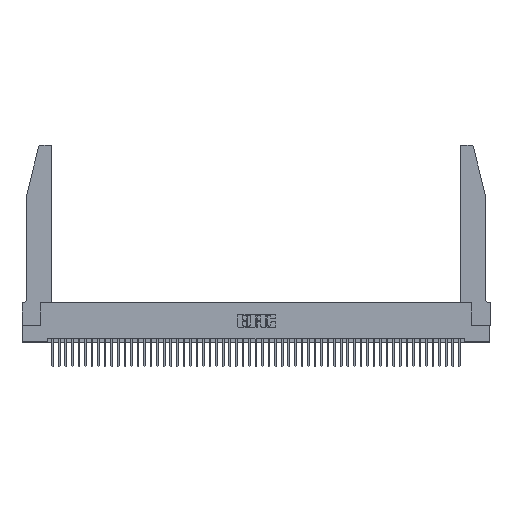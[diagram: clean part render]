
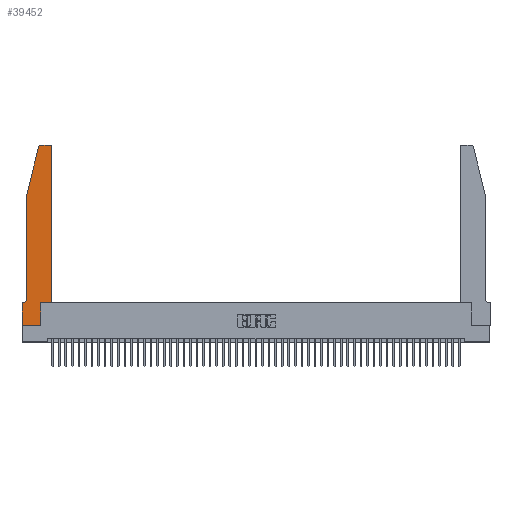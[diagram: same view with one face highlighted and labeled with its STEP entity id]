
A CAD part, top view. The second image highlights one B-rep face of the part: STEP entity #39452.
In plain terms, the highlighted planar face has unit normal (0, 0, 1).
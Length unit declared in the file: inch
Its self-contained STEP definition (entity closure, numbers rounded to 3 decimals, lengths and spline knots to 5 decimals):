
#424 = LINE ( 'NONE', #24426, #38902 ) ;
#468 = VECTOR ( 'NONE', #25666, 39.37008 ) ;
#502 = AXIS2_PLACEMENT_3D ( 'NONE', #27071, #50351, #46513 ) ;
#571 = VERTEX_POINT ( 'NONE', #48811 ) ;
#1234 = CARTESIAN_POINT ( 'NONE',  ( 0.2605, 2.75, 0.37 ) ) ;
#1330 = VECTOR ( 'NONE', #19724, 39.37008 ) ;
#1846 = DIRECTION ( 'NONE',  ( 0., -1., 0. ) ) ;
#2422 = EDGE_CURVE ( 'NONE', #31493, #47907, #22815, .T. ) ;
#2819 = VECTOR ( 'NONE', #23073, 39.37008 ) ;
#2908 = CARTESIAN_POINT ( 'NONE',  ( 0., 0., 0.37 ) ) ;
#2964 = ORIENTED_EDGE ( 'NONE', *, *, #2422, .T. ) ;
#2999 = EDGE_CURVE ( 'NONE', #46961, #31018, #424, .T. ) ;
#3189 = CARTESIAN_POINT ( 'NONE',  ( 0.284, 2.75, 0.37 ) ) ;
#3436 = CARTESIAN_POINT ( 'NONE',  ( 0.2865, 0.35, 0.37 ) ) ;
#4125 = CIRCLE ( 'NONE', #18013, 0.03 ) ;
#4364 = CIRCLE ( 'NONE', #39853, 0.03 ) ;
#5432 = ORIENTED_EDGE ( 'NONE', *, *, #38660, .T. ) ;
#5646 = EDGE_CURVE ( 'NONE', #20788, #46961, #23670, .T. ) ;
#6351 = VECTOR ( 'NONE', #25296, 39.37008 ) ;
#6635 = PLANE ( 'NONE',  #33865 ) ;
#7294 = CARTESIAN_POINT ( 'NONE',  ( 0.0055, 0.35, 0.37 ) ) ;
#7648 = VECTOR ( 'NONE', #30325, 39.37008 ) ;
#7833 = ORIENTED_EDGE ( 'NONE', *, *, #25196, .T. ) ;
#7897 = ORIENTED_EDGE ( 'NONE', *, *, #5646, .T. ) ;
#8317 = CARTESIAN_POINT ( 'NONE',  ( 0.2865, 0.35, 0.37 ) ) ;
#9077 = ORIENTED_EDGE ( 'NONE', *, *, #36775, .T. ) ;
#9507 = EDGE_CURVE ( 'NONE', #31018, #13375, #33835, .T. ) ;
#9522 = CARTESIAN_POINT ( 'NONE',  ( 0.0755, 2., 0.37 ) ) ;
#10010 = ORIENTED_EDGE ( 'NONE', *, *, #2999, .T. ) ;
#10829 = CARTESIAN_POINT ( 'NONE',  ( 0., 0.35, 0.37 ) ) ;
#11681 = VERTEX_POINT ( 'NONE', #48966 ) ;
#11973 = VERTEX_POINT ( 'NONE', #2908 ) ;
#12376 = ORIENTED_EDGE ( 'NONE', *, *, #41454, .T. ) ;
#13375 = VERTEX_POINT ( 'NONE', #30405 ) ;
#13486 = ORIENTED_EDGE ( 'NONE', *, *, #9507, .T. ) ;
#14643 = DIRECTION ( 'NONE',  ( 1., 0., 0. ) ) ;
#15392 = ORIENTED_EDGE ( 'NONE', *, *, #37172, .T. ) ;
#15480 = CARTESIAN_POINT ( 'NONE',  ( 0.284, 2.72, 0.37 ) ) ;
#15869 = CARTESIAN_POINT ( 'NONE',  ( 0., 0., 0.37 ) ) ;
#16995 = DIRECTION ( 'NONE',  ( 1., 0., 0. ) ) ;
#18013 = AXIS2_PLACEMENT_3D ( 'NONE', #24133, #36294, #28321 ) ;
#18728 = VERTEX_POINT ( 'NONE', #3189 ) ;
#19566 = VECTOR ( 'NONE', #28675, 39.37008 ) ;
#19724 = DIRECTION ( 'NONE',  ( 0., 1., 0. ) ) ;
#20788 = VERTEX_POINT ( 'NONE', #32162 ) ;
#21503 = CARTESIAN_POINT ( 'NONE',  ( 0.0755, 2., 0.37 ) ) ;
#21998 = CARTESIAN_POINT ( 'NONE',  ( 0.25487, 2.72718, 0.37 ) ) ;
#22579 = DIRECTION ( 'NONE',  ( 0., 0., 1. ) ) ;
#22815 = LINE ( 'NONE', #21503, #468 ) ;
#23073 = DIRECTION ( 'NONE',  ( 0., 1., 0. ) ) ;
#23145 = LINE ( 'NONE', #50287, #7648 ) ;
#23670 = LINE ( 'NONE', #8317, #1330 ) ;
#23831 = CARTESIAN_POINT ( 'NONE',  ( 0., 0.35, 0.37 ) ) ;
#24133 = CARTESIAN_POINT ( 'NONE',  ( 0.4205, 2.72, 0.37 ) ) ;
#24426 = CARTESIAN_POINT ( 'NONE',  ( 0.4505, 0.35, 0.37 ) ) ;
#24774 = ORIENTED_EDGE ( 'NONE', *, *, #33399, .T. ) ;
#24796 = VECTOR ( 'NONE', #1846, 39.37008 ) ;
#25196 = EDGE_CURVE ( 'NONE', #18728, #31493, #4364, .T. ) ;
#25296 = DIRECTION ( 'NONE',  ( 1., 0., 0. ) ) ;
#25666 = DIRECTION ( 'NONE',  ( -0.239, -0.971, 0. ) ) ;
#26063 = EDGE_LOOP ( 'NONE', ( #12376, #7833, #2964, #5432, #48761, #9077, #15392, #24774, #7897, #10010, #13486, #45482 ) ) ;
#26932 = DIRECTION ( 'NONE',  ( 0., 0., 1. ) ) ;
#27071 = CARTESIAN_POINT ( 'NONE',  ( 0.0055, 0.42, 0.37 ) ) ;
#27257 = CARTESIAN_POINT ( 'NONE',  ( 0.4505, 0.35, 0.37 ) ) ;
#28321 = DIRECTION ( 'NONE',  ( 1., 0., 0. ) ) ;
#28675 = DIRECTION ( 'NONE',  ( -1., 0., 0. ) ) ;
#29334 = VERTEX_POINT ( 'NONE', #7294 ) ;
#30163 = LINE ( 'NONE', #1234, #19566 ) ;
#30297 = FACE_OUTER_BOUND ( 'NONE', #26063, .T. ) ;
#30325 = DIRECTION ( 'NONE',  ( -1., 0., 0. ) ) ;
#30405 = CARTESIAN_POINT ( 'NONE',  ( 0.4505, 2.72, 0.37 ) ) ;
#30602 = VECTOR ( 'NONE', #51102, 39.37008 ) ;
#31018 = VERTEX_POINT ( 'NONE', #50860 ) ;
#31493 = VERTEX_POINT ( 'NONE', #21998 ) ;
#32162 = CARTESIAN_POINT ( 'NONE',  ( 0.2865, 0., 0.37 ) ) ;
#32775 = CIRCLE ( 'NONE', #502, 0.07 ) ;
#33399 = EDGE_CURVE ( 'NONE', #11973, #20788, #43574, .T. ) ;
#33442 = CARTESIAN_POINT ( 'NONE',  ( 0., 0., 0.37 ) ) ;
#33835 = LINE ( 'NONE', #27257, #2819 ) ;
#33865 = AXIS2_PLACEMENT_3D ( 'NONE', #10829, #22579, #14643 ) ;
#36294 = DIRECTION ( 'NONE',  ( 0., 0., 1. ) ) ;
#36319 = EDGE_CURVE ( 'NONE', #11681, #29334, #32775, .T. ) ;
#36775 = EDGE_CURVE ( 'NONE', #29334, #44489, #23145, .T. ) ;
#37172 = EDGE_CURVE ( 'NONE', #44489, #11973, #37437, .T. ) ;
#37437 = LINE ( 'NONE', #15869, #30602 ) ;
#38660 = EDGE_CURVE ( 'NONE', #47907, #11681, #39075, .T. ) ;
#38902 = VECTOR ( 'NONE', #16995, 39.37008 ) ;
#39075 = LINE ( 'NONE', #9522, #24796 ) ;
#39452 = ADVANCED_FACE ( 'NONE', ( #30297 ), #6635, .T. ) ;
#39853 = AXIS2_PLACEMENT_3D ( 'NONE', #15480, #26932, #50878 ) ;
#41231 = EDGE_CURVE ( 'NONE', #13375, #571, #4125, .T. ) ;
#41454 = EDGE_CURVE ( 'NONE', #571, #18728, #30163, .T. ) ;
#43574 = LINE ( 'NONE', #33442, #6351 ) ;
#44489 = VERTEX_POINT ( 'NONE', #23831 ) ;
#45482 = ORIENTED_EDGE ( 'NONE', *, *, #41231, .T. ) ;
#46513 = DIRECTION ( 'NONE',  ( -1., 0., 0. ) ) ;
#46961 = VERTEX_POINT ( 'NONE', #3436 ) ;
#47907 = VERTEX_POINT ( 'NONE', #49522 ) ;
#48761 = ORIENTED_EDGE ( 'NONE', *, *, #36319, .T. ) ;
#48811 = CARTESIAN_POINT ( 'NONE',  ( 0.4205, 2.75, 0.37 ) ) ;
#48966 = CARTESIAN_POINT ( 'NONE',  ( 0.0755, 0.42, 0.37 ) ) ;
#49522 = CARTESIAN_POINT ( 'NONE',  ( 0.0755, 2., 0.37 ) ) ;
#50287 = CARTESIAN_POINT ( 'NONE',  ( 0.0755, 0.35, 0.37 ) ) ;
#50351 = DIRECTION ( 'NONE',  ( 0., 0., -1. ) ) ;
#50860 = CARTESIAN_POINT ( 'NONE',  ( 0.4505, 0.35, 0.37 ) ) ;
#50878 = DIRECTION ( 'NONE',  ( 1., 0., 0. ) ) ;
#51102 = DIRECTION ( 'NONE',  ( 0., -1., 0. ) ) ;
